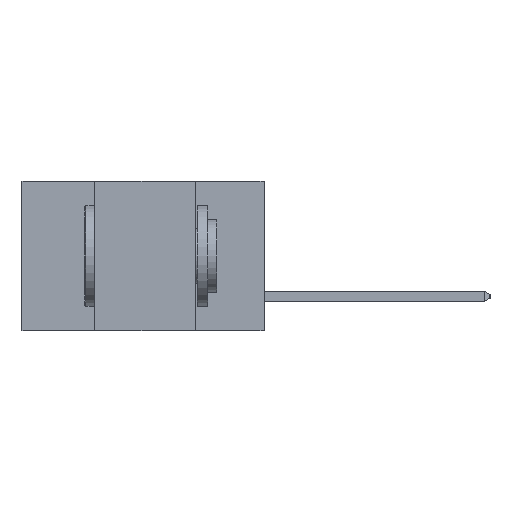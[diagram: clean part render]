
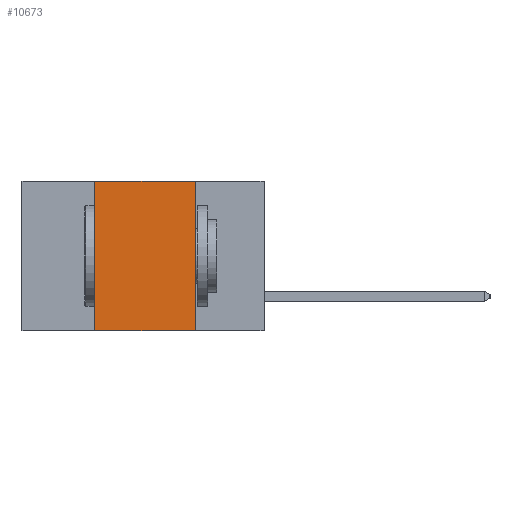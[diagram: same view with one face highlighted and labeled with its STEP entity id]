
A CAD part, left-side view. The second image highlights one B-rep face of the part: STEP entity #10673.
In plain terms, the highlighted planar face has unit normal (-1, 0, 0).
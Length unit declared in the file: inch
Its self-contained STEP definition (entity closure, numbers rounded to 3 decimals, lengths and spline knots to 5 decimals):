
#16 = CARTESIAN_POINT ( 'NONE',  ( 0., 0.17, -0.37 ) ) ;
#823 = DIRECTION ( 'NONE',  ( 0., 0., -1. ) ) ;
#1414 = LINE ( 'NONE', #9029, #6917 ) ;
#1830 = FACE_OUTER_BOUND ( 'NONE', #6518, .T. ) ;
#2222 = VERTEX_POINT ( 'NONE', #13053 ) ;
#2461 = VERTEX_POINT ( 'NONE', #11274 ) ;
#3914 = EDGE_CURVE ( 'NONE', #2222, #10998, #6151, .T. ) ;
#3975 = EDGE_CURVE ( 'NONE', #4348, #2222, #8196, .T. ) ;
#4026 = ORIENTED_EDGE ( 'NONE', *, *, #4062, .T. ) ;
#4038 = EDGE_CURVE ( 'NONE', #2461, #4348, #7551, .T. ) ;
#4062 = EDGE_CURVE ( 'NONE', #2461, #10998, #1414, .T. ) ;
#4348 = VERTEX_POINT ( 'NONE', #6478 ) ;
#4369 = PLANE ( 'NONE',  #13364 ) ;
#6151 = LINE ( 'NONE', #11414, #6458 ) ;
#6458 = VECTOR ( 'NONE', #9835, 39.37008 ) ;
#6478 = CARTESIAN_POINT ( 'NONE',  ( 0., 0.42, 0. ) ) ;
#6518 = EDGE_LOOP ( 'NONE', ( #10468, #12959, #8795, #4026 ) ) ;
#6917 = VECTOR ( 'NONE', #8803, 39.37008 ) ;
#7440 = DIRECTION ( 'NONE',  ( 1., 0., 0. ) ) ;
#7551 = LINE ( 'NONE', #7960, #9895 ) ;
#7712 = DIRECTION ( 'NONE',  ( 0., 0., 1. ) ) ;
#7960 = CARTESIAN_POINT ( 'NONE',  ( 0., 0.42, -0.37 ) ) ;
#8017 = CARTESIAN_POINT ( 'NONE',  ( 0., 0.6, 0. ) ) ;
#8196 = LINE ( 'NONE', #8017, #12982 ) ;
#8795 = ORIENTED_EDGE ( 'NONE', *, *, #4038, .F. ) ;
#8803 = DIRECTION ( 'NONE',  ( 0., -1., 0. ) ) ;
#8885 = DIRECTION ( 'NONE',  ( 0., -1., 0. ) ) ;
#9029 = CARTESIAN_POINT ( 'NONE',  ( 0., 0.6, -0.37 ) ) ;
#9396 = CARTESIAN_POINT ( 'NONE',  ( 0., 0.6, 0. ) ) ;
#9835 = DIRECTION ( 'NONE',  ( 0., 0., -1. ) ) ;
#9895 = VECTOR ( 'NONE', #7712, 39.37008 ) ;
#10468 = ORIENTED_EDGE ( 'NONE', *, *, #3914, .F. ) ;
#10673 = ADVANCED_FACE ( 'NONE', ( #1830 ), #4369, .F. ) ;
#10998 = VERTEX_POINT ( 'NONE', #16 ) ;
#11274 = CARTESIAN_POINT ( 'NONE',  ( 0., 0.42, -0.37 ) ) ;
#11414 = CARTESIAN_POINT ( 'NONE',  ( 0., 0.17, -0.37 ) ) ;
#12959 = ORIENTED_EDGE ( 'NONE', *, *, #3975, .F. ) ;
#12982 = VECTOR ( 'NONE', #8885, 39.37008 ) ;
#13053 = CARTESIAN_POINT ( 'NONE',  ( 0., 0.17, 0. ) ) ;
#13364 = AXIS2_PLACEMENT_3D ( 'NONE', #9396, #7440, #823 ) ;
